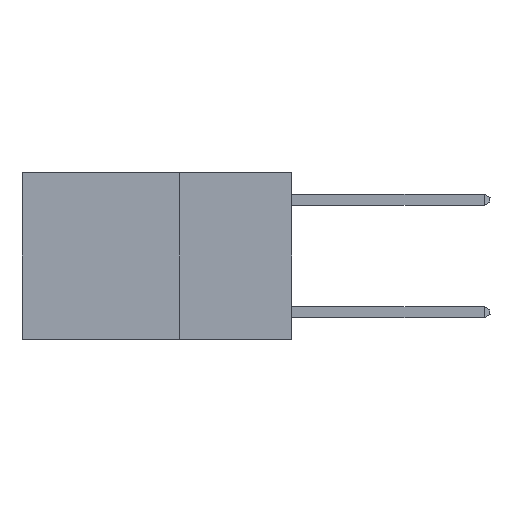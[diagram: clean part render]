
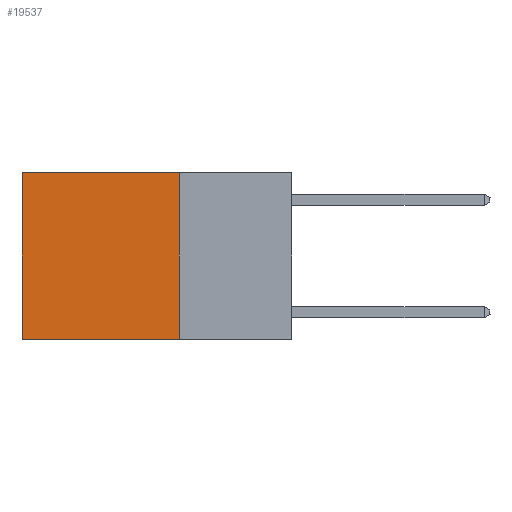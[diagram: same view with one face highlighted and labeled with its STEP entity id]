
A CAD part, left-side view. The second image highlights one B-rep face of the part: STEP entity #19537.
In plain terms, the highlighted planar face has unit normal (-1, 0, 0).
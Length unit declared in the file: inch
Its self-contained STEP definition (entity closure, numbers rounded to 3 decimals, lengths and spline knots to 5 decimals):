
#1 = LINE ( 'NONE', #11148, #8122 ) ;
#1822 = VERTEX_POINT ( 'NONE', #12176 ) ;
#2388 = VECTOR ( 'NONE', #20230, 39.37008 ) ;
#2981 = ORIENTED_EDGE ( 'NONE', *, *, #7256, .T. ) ;
#4230 = CARTESIAN_POINT ( 'NONE',  ( 0.2625, 0.25, -0.37 ) ) ;
#4721 = EDGE_CURVE ( 'NONE', #7959, #1822, #1, .T. ) ;
#6735 = VERTEX_POINT ( 'NONE', #15094 ) ;
#6772 = ORIENTED_EDGE ( 'NONE', *, *, #20949, .F. ) ;
#7256 = EDGE_CURVE ( 'NONE', #1822, #6735, #7649, .T. ) ;
#7472 = DIRECTION ( 'NONE',  ( 0., 1., 0. ) ) ;
#7649 = LINE ( 'NONE', #16955, #18281 ) ;
#7762 = DIRECTION ( 'NONE',  ( 0., 0., -1. ) ) ;
#7959 = VERTEX_POINT ( 'NONE', #23000 ) ;
#8009 = FACE_OUTER_BOUND ( 'NONE', #21681, .T. ) ;
#8122 = VECTOR ( 'NONE', #7472, 39.37008 ) ;
#9038 = EDGE_CURVE ( 'NONE', #7959, #17286, #22006, .T. ) ;
#9158 = CARTESIAN_POINT ( 'NONE',  ( 0.2625, 0.25, 0. ) ) ;
#9844 = ORIENTED_EDGE ( 'NONE', *, *, #9038, .F. ) ;
#11148 = CARTESIAN_POINT ( 'NONE',  ( 0.2625, 0.25, 0. ) ) ;
#12176 = CARTESIAN_POINT ( 'NONE',  ( 0.2625, 0.6, 0. ) ) ;
#15094 = CARTESIAN_POINT ( 'NONE',  ( 0.2625, 0.6, -0.37 ) ) ;
#16955 = CARTESIAN_POINT ( 'NONE',  ( 0.2625, 0.6, 0. ) ) ;
#16968 = DIRECTION ( 'NONE',  ( 1., 0., 0. ) ) ;
#17286 = VERTEX_POINT ( 'NONE', #4230 ) ;
#17717 = DIRECTION ( 'NONE',  ( 0., 1., 0. ) ) ;
#18281 = VECTOR ( 'NONE', #7762, 39.37008 ) ;
#19537 = ADVANCED_FACE ( 'NONE', ( #8009 ), #20727, .F. ) ;
#19836 = VECTOR ( 'NONE', #17717, 39.37008 ) ;
#20230 = DIRECTION ( 'NONE',  ( 0., 0., -1. ) ) ;
#20617 = DIRECTION ( 'NONE',  ( 0., 0., -1. ) ) ;
#20727 = PLANE ( 'NONE',  #22785 ) ;
#20949 = EDGE_CURVE ( 'NONE', #17286, #6735, #21612, .T. ) ;
#21612 = LINE ( 'NONE', #23142, #19836 ) ;
#21681 = EDGE_LOOP ( 'NONE', ( #2981, #6772, #9844, #22430 ) ) ;
#22006 = LINE ( 'NONE', #9158, #2388 ) ;
#22374 = CARTESIAN_POINT ( 'NONE',  ( 0.2625, 0.25, 0. ) ) ;
#22430 = ORIENTED_EDGE ( 'NONE', *, *, #4721, .T. ) ;
#22785 = AXIS2_PLACEMENT_3D ( 'NONE', #22374, #16968, #20617 ) ;
#23000 = CARTESIAN_POINT ( 'NONE',  ( 0.2625, 0.25, 0. ) ) ;
#23142 = CARTESIAN_POINT ( 'NONE',  ( 0.2625, 0.25, -0.37 ) ) ;
